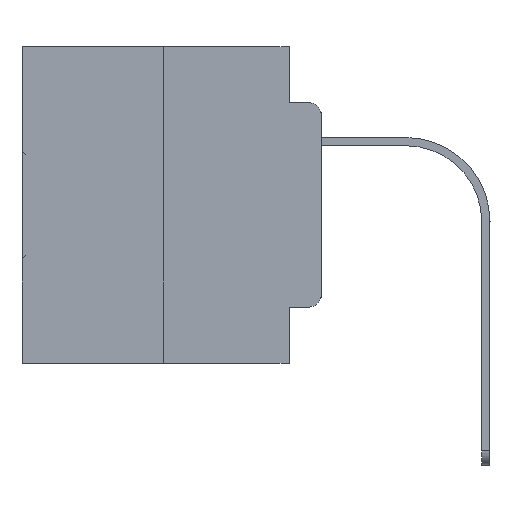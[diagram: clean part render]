
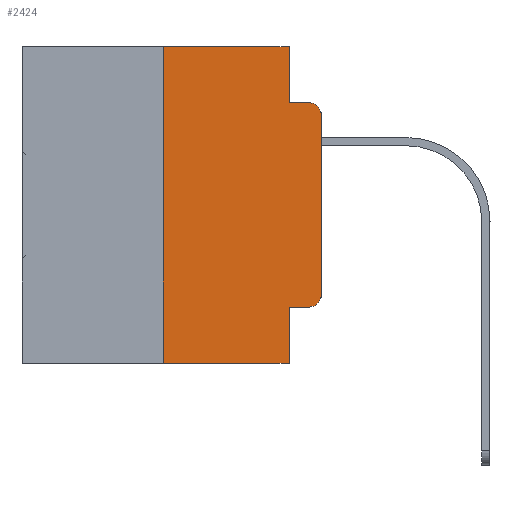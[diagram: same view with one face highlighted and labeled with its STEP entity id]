
A CAD part, left-side view. The second image highlights one B-rep face of the part: STEP entity #2424.
In plain terms, the highlighted planar face has unit normal (-1, 0, 0).
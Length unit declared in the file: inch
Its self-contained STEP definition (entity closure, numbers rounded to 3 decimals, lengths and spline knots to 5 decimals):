
#555 = CIRCLE ( 'NONE', #10418, 0.02 ) ;
#652 = ORIENTED_EDGE ( 'NONE', *, *, #18194, .F. ) ;
#767 = CARTESIAN_POINT ( 'NONE',  ( 0., 0.473, 0. ) ) ;
#916 = FACE_OUTER_BOUND ( 'NONE', #30789, .T. ) ;
#1985 = CARTESIAN_POINT ( 'NONE',  ( 0., 0.25, -0.5 ) ) ;
#2057 = VECTOR ( 'NONE', #17000, 39.37008 ) ;
#2424 = ADVANCED_FACE ( 'NONE', ( #916 ), #7901, .F. ) ;
#2579 = ORIENTED_EDGE ( 'NONE', *, *, #23441, .T. ) ;
#2673 = VECTOR ( 'NONE', #27923, 39.37008 ) ;
#2903 = CARTESIAN_POINT ( 'NONE',  ( 0., 0.25, 0. ) ) ;
#3613 = EDGE_CURVE ( 'NONE', #25343, #17564, #5041, .T. ) ;
#3637 = VERTEX_POINT ( 'NONE', #2903 ) ;
#4113 = LINE ( 'NONE', #11650, #23858 ) ;
#5041 = LINE ( 'NONE', #17565, #28177 ) ;
#5401 = VERTEX_POINT ( 'NONE', #20932 ) ;
#5598 = LINE ( 'NONE', #24822, #2673 ) ;
#6872 = DIRECTION ( 'NONE',  ( 0., -1., 0. ) ) ;
#7312 = EDGE_CURVE ( 'NONE', #25103, #13744, #26779, .T. ) ;
#7504 = DIRECTION ( 'NONE',  ( -1., 0., 0. ) ) ;
#7684 = CARTESIAN_POINT ( 'NONE',  ( 0., 0.02, -0.1085 ) ) ;
#7901 = PLANE ( 'NONE',  #26598 ) ;
#8018 = CARTESIAN_POINT ( 'NONE',  ( 0., 0.473, 0. ) ) ;
#8663 = DIRECTION ( 'NONE',  ( 0., -1., 0. ) ) ;
#8803 = EDGE_CURVE ( 'NONE', #3637, #18018, #17779, .T. ) ;
#9216 = CARTESIAN_POINT ( 'NONE',  ( 0., 0., -0.1085 ) ) ;
#9520 = LINE ( 'NONE', #26790, #2057 ) ;
#10418 = AXIS2_PLACEMENT_3D ( 'NONE', #22153, #7504, #27518 ) ;
#10673 = EDGE_CURVE ( 'NONE', #5401, #21727, #9520, .T. ) ;
#11317 = CARTESIAN_POINT ( 'NONE',  ( 0., 0.051, -0.0885 ) ) ;
#11650 = CARTESIAN_POINT ( 'NONE',  ( 0., 0.473, -0.5 ) ) ;
#11777 = EDGE_CURVE ( 'NONE', #21727, #13744, #12074, .T. ) ;
#12074 = CIRCLE ( 'NONE', #21416, 0.02 ) ;
#12524 = ORIENTED_EDGE ( 'NONE', *, *, #25919, .F. ) ;
#13230 = VECTOR ( 'NONE', #25914, 39.37008 ) ;
#13320 = DIRECTION ( 'NONE',  ( 1., 0., 0. ) ) ;
#13744 = VERTEX_POINT ( 'NONE', #29826 ) ;
#14132 = VECTOR ( 'NONE', #18165, 39.37008 ) ;
#14341 = CARTESIAN_POINT ( 'NONE',  ( 0., 0.02, -0.4115 ) ) ;
#14453 = CARTESIAN_POINT ( 'NONE',  ( 0., 0.051, 0. ) ) ;
#17000 = DIRECTION ( 'NONE',  ( 0., 0., 1. ) ) ;
#17424 = DIRECTION ( 'NONE',  ( 0., 0., -1. ) ) ;
#17564 = VERTEX_POINT ( 'NONE', #26845 ) ;
#17565 = CARTESIAN_POINT ( 'NONE',  ( 0., 0.051, 0. ) ) ;
#17638 = VERTEX_POINT ( 'NONE', #14341 ) ;
#17779 = LINE ( 'NONE', #8018, #13230 ) ;
#18017 = CARTESIAN_POINT ( 'NONE',  ( 0., 0.25, 0. ) ) ;
#18018 = VERTEX_POINT ( 'NONE', #14453 ) ;
#18028 = ORIENTED_EDGE ( 'NONE', *, *, #7312, .F. ) ;
#18165 = DIRECTION ( 'NONE',  ( 0., 0., 1. ) ) ;
#18194 = EDGE_CURVE ( 'NONE', #18018, #25103, #5598, .T. ) ;
#18911 = CARTESIAN_POINT ( 'NONE',  ( 0., 0.051, -0.4115 ) ) ;
#19195 = VECTOR ( 'NONE', #6872, 39.37008 ) ;
#20932 = CARTESIAN_POINT ( 'NONE',  ( 0., 0., -0.3915 ) ) ;
#21229 = ORIENTED_EDGE ( 'NONE', *, *, #11777, .T. ) ;
#21416 = AXIS2_PLACEMENT_3D ( 'NONE', #7684, #30496, #27561 ) ;
#21558 = DIRECTION ( 'NONE',  ( 0., -1., 0. ) ) ;
#21727 = VERTEX_POINT ( 'NONE', #9216 ) ;
#22153 = CARTESIAN_POINT ( 'NONE',  ( 0., 0.02, -0.3915 ) ) ;
#22742 = LINE ( 'NONE', #18017, #14132 ) ;
#23372 = DIRECTION ( 'NONE',  ( 0., 0., -1. ) ) ;
#23441 = EDGE_CURVE ( 'NONE', #23497, #17564, #4113, .T. ) ;
#23497 = VERTEX_POINT ( 'NONE', #1985 ) ;
#23858 = VECTOR ( 'NONE', #21558, 39.37008 ) ;
#23867 = EDGE_CURVE ( 'NONE', #25343, #17638, #24281, .T. ) ;
#24281 = LINE ( 'NONE', #18911, #29073 ) ;
#24822 = CARTESIAN_POINT ( 'NONE',  ( 0., 0.051, 0. ) ) ;
#25103 = VERTEX_POINT ( 'NONE', #30860 ) ;
#25316 = EDGE_CURVE ( 'NONE', #17638, #5401, #555, .T. ) ;
#25343 = VERTEX_POINT ( 'NONE', #30122 ) ;
#25914 = DIRECTION ( 'NONE',  ( 0., -1., 0. ) ) ;
#25919 = EDGE_CURVE ( 'NONE', #23497, #3637, #22742, .T. ) ;
#26598 = AXIS2_PLACEMENT_3D ( 'NONE', #767, #13320, #23372 ) ;
#26779 = LINE ( 'NONE', #11317, #19195 ) ;
#26790 = CARTESIAN_POINT ( 'NONE',  ( 0., 0., 0. ) ) ;
#26845 = CARTESIAN_POINT ( 'NONE',  ( 0., 0.051, -0.5 ) ) ;
#27048 = ORIENTED_EDGE ( 'NONE', *, *, #3613, .F. ) ;
#27518 = DIRECTION ( 'NONE',  ( 0., 0., -1. ) ) ;
#27561 = DIRECTION ( 'NONE',  ( 0., 0., -1. ) ) ;
#27923 = DIRECTION ( 'NONE',  ( 0., 0., -1. ) ) ;
#28177 = VECTOR ( 'NONE', #17424, 39.37008 ) ;
#29073 = VECTOR ( 'NONE', #8663, 39.37008 ) ;
#29124 = ORIENTED_EDGE ( 'NONE', *, *, #10673, .T. ) ;
#29826 = CARTESIAN_POINT ( 'NONE',  ( 0., 0.02, -0.0885 ) ) ;
#30122 = CARTESIAN_POINT ( 'NONE',  ( 0., 0.051, -0.4115 ) ) ;
#30233 = ORIENTED_EDGE ( 'NONE', *, *, #23867, .T. ) ;
#30496 = DIRECTION ( 'NONE',  ( -1., 0., 0. ) ) ;
#30789 = EDGE_LOOP ( 'NONE', ( #29124, #21229, #18028, #652, #31359, #12524, #2579, #27048, #30233, #31888 ) ) ;
#30860 = CARTESIAN_POINT ( 'NONE',  ( 0., 0.051, -0.0885 ) ) ;
#31359 = ORIENTED_EDGE ( 'NONE', *, *, #8803, .F. ) ;
#31888 = ORIENTED_EDGE ( 'NONE', *, *, #25316, .T. ) ;
